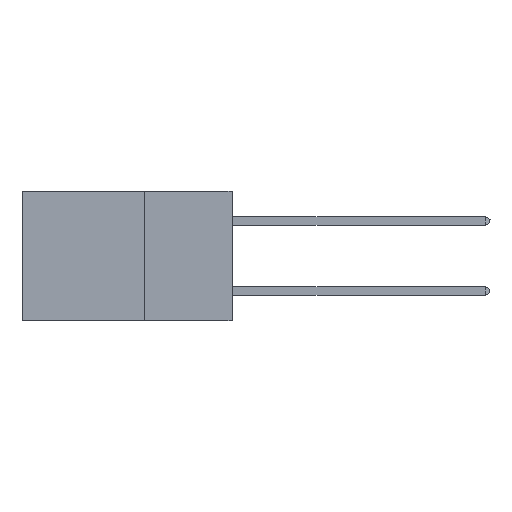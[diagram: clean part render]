
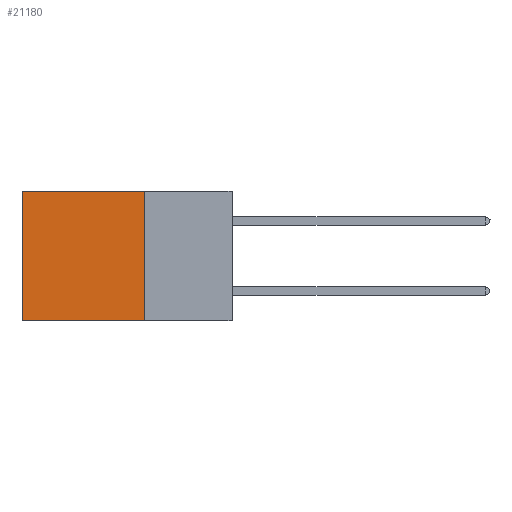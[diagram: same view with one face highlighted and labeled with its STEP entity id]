
A CAD part, left-side view. The second image highlights one B-rep face of the part: STEP entity #21180.
In plain terms, the highlighted planar face has unit normal (-1, 0, 0).
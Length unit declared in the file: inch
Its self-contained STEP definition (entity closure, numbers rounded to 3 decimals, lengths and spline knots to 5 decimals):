
#992 = VERTEX_POINT ( 'NONE', #34799 ) ;
#2297 = LINE ( 'NONE', #13256, #3574 ) ;
#2936 = ORIENTED_EDGE ( 'NONE', *, *, #33665, .T. ) ;
#3059 = EDGE_CURVE ( 'NONE', #34676, #12199, #27150, .T. ) ;
#3574 = VECTOR ( 'NONE', #26580, 39.37008 ) ;
#4651 = CARTESIAN_POINT ( 'NONE',  ( 0.2875, 0.25, 0. ) ) ;
#5358 = DIRECTION ( 'NONE',  ( 0., 0., -1. ) ) ;
#6093 = CARTESIAN_POINT ( 'NONE',  ( 0.2875, 0.6, -0.37 ) ) ;
#8335 = ORIENTED_EDGE ( 'NONE', *, *, #3059, .F. ) ;
#10408 = CARTESIAN_POINT ( 'NONE',  ( 0.2875, 0.6, 0. ) ) ;
#10829 = CARTESIAN_POINT ( 'NONE',  ( 0.2875, 0.25, -0.37 ) ) ;
#12199 = VERTEX_POINT ( 'NONE', #6093 ) ;
#13074 = EDGE_LOOP ( 'NONE', ( #2936, #8335, #20029, #33817 ) ) ;
#13256 = CARTESIAN_POINT ( 'NONE',  ( 0.2875, 0.25, 0. ) ) ;
#13439 = EDGE_CURVE ( 'NONE', #992, #34676, #2297, .T. ) ;
#13582 = DIRECTION ( 'NONE',  ( 1., 0., 0. ) ) ;
#14501 = DIRECTION ( 'NONE',  ( 0., 0., -1. ) ) ;
#17055 = CARTESIAN_POINT ( 'NONE',  ( 0.2875, 0.6, 0. ) ) ;
#17791 = CARTESIAN_POINT ( 'NONE',  ( 0.2875, 0.25, 0. ) ) ;
#18534 = FACE_OUTER_BOUND ( 'NONE', #13074, .T. ) ;
#19697 = DIRECTION ( 'NONE',  ( 0., 1., 0. ) ) ;
#20029 = ORIENTED_EDGE ( 'NONE', *, *, #13439, .F. ) ;
#20428 = VERTEX_POINT ( 'NONE', #10408 ) ;
#21180 = ADVANCED_FACE ( 'NONE', ( #18534 ), #29622, .F. ) ;
#22426 = LINE ( 'NONE', #17791, #34831 ) ;
#25438 = CARTESIAN_POINT ( 'NONE',  ( 0.2875, 0.25, -0.37 ) ) ;
#26580 = DIRECTION ( 'NONE',  ( 0., 0., -1. ) ) ;
#26958 = VECTOR ( 'NONE', #31070, 39.37008 ) ;
#27150 = LINE ( 'NONE', #25438, #26958 ) ;
#28676 = EDGE_CURVE ( 'NONE', #992, #20428, #22426, .T. ) ;
#28931 = AXIS2_PLACEMENT_3D ( 'NONE', #4651, #13582, #5358 ) ;
#29622 = PLANE ( 'NONE',  #28931 ) ;
#31070 = DIRECTION ( 'NONE',  ( 0., 1., 0. ) ) ;
#32725 = VECTOR ( 'NONE', #14501, 39.37008 ) ;
#33665 = EDGE_CURVE ( 'NONE', #20428, #12199, #33810, .T. ) ;
#33810 = LINE ( 'NONE', #17055, #32725 ) ;
#33817 = ORIENTED_EDGE ( 'NONE', *, *, #28676, .T. ) ;
#34676 = VERTEX_POINT ( 'NONE', #10829 ) ;
#34799 = CARTESIAN_POINT ( 'NONE',  ( 0.2875, 0.25, 0. ) ) ;
#34831 = VECTOR ( 'NONE', #19697, 39.37008 ) ;
